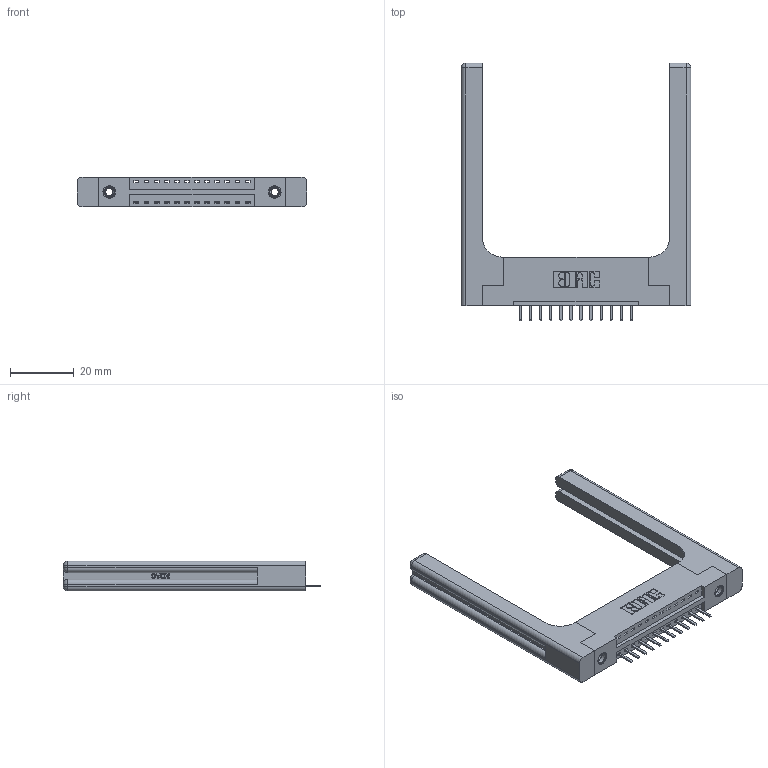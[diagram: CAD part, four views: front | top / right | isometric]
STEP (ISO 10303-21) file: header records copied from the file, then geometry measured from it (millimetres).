
FILE_DESCRIPTION (( 'STEP AP203' ), '1' );
FILE_NAME ('396-012-520-158.STEP', '2019-10-26T15:15:08', ( '' ), ( '' ), 'SwSTEP 2.0', 'SolidWorks 2016', '' );
FILE_SCHEMA (( 'CONFIG_CONTROL_DESIGN' ));
Length unit declared in the file: inch
Products named in the file (5): 346 Part_Flush Mounting Lugs - 0.156 Dia-TH; 346-220-058_345-220-058; 345-292-001_345-293-120; 396-012-520-158; 345-250-001_345-250-001-102
Assembly tree (17 placements, depth 2):
  396-012-520-158
    346 Part_Flush Mounting Lugs - 0.156 Dia-TH
    345-292-001_345-293-120  x12
    345-250-001_345-250-001-102  x2
    346-220-058_345-220-058  x2
Bounding box: 72.16 x 80.98 x 9.4 mm (x, y, z)
Volume: 14184.6 mm3; surface area: 13062.5 mm2
Topology: 17 solids, 17 shells, 1122 faces, 3203 edges, 2082 vertices
Faces by surface type: plane 728, cylinder 334, bspline 36, cone 12, sphere 8, torus 4
Entity records: 16782 total; most frequent: CARTESIAN_POINT 3877, ORIENTED_EDGE 2608, DIRECTION 2376, EDGE_CURVE 1304, LINE 1028, VECTOR 1028, VERTEX_POINT 858, AXIS2_PLACEMENT_3D 674
